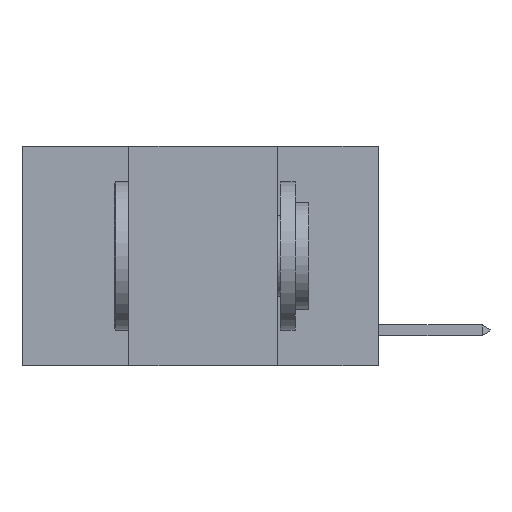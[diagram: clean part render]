
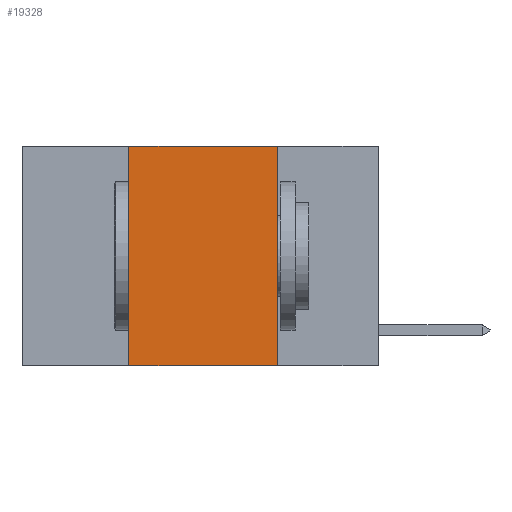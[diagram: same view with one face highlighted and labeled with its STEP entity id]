
A CAD part, left-side view. The second image highlights one B-rep face of the part: STEP entity #19328.
In plain terms, the highlighted planar face has unit normal (-1, 0, 0).
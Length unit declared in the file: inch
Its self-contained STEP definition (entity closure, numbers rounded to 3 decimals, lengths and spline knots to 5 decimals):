
#16 = EDGE_LOOP ( 'NONE', ( #15866, #12342, #7933, #7472 ) ) ;
#1249 = VECTOR ( 'NONE', #18999, 39.37008 ) ;
#1775 = LINE ( 'NONE', #7853, #6517 ) ;
#1973 = DIRECTION ( 'NONE',  ( 0., -1., 0. ) ) ;
#2403 = LINE ( 'NONE', #3987, #1249 ) ;
#3654 = FACE_OUTER_BOUND ( 'NONE', #16, .T. ) ;
#3766 = VERTEX_POINT ( 'NONE', #7858 ) ;
#3987 = CARTESIAN_POINT ( 'NONE',  ( 0., 0.6, 0. ) ) ;
#4887 = VERTEX_POINT ( 'NONE', #8288 ) ;
#5133 = DIRECTION ( 'NONE',  ( 0., 0., -1. ) ) ;
#5409 = DIRECTION ( 'NONE',  ( 0., 0., -1. ) ) ;
#5807 = DIRECTION ( 'NONE',  ( 0., 0., 1. ) ) ;
#6517 = VECTOR ( 'NONE', #1973, 39.37008 ) ;
#7255 = VECTOR ( 'NONE', #5807, 39.37008 ) ;
#7472 = ORIENTED_EDGE ( 'NONE', *, *, #8326, .T. ) ;
#7630 = VECTOR ( 'NONE', #5409, 39.37008 ) ;
#7853 = CARTESIAN_POINT ( 'NONE',  ( 0., 0.6, -0.37 ) ) ;
#7858 = CARTESIAN_POINT ( 'NONE',  ( 0., 0.17, -0.37 ) ) ;
#7933 = ORIENTED_EDGE ( 'NONE', *, *, #12472, .F. ) ;
#8288 = CARTESIAN_POINT ( 'NONE',  ( 0., 0.17, 0. ) ) ;
#8326 = EDGE_CURVE ( 'NONE', #10758, #3766, #1775, .T. ) ;
#8626 = LINE ( 'NONE', #11399, #7630 ) ;
#10227 = CARTESIAN_POINT ( 'NONE',  ( 0., 0.42, -0.37 ) ) ;
#10758 = VERTEX_POINT ( 'NONE', #10227 ) ;
#11399 = CARTESIAN_POINT ( 'NONE',  ( 0., 0.17, 0. ) ) ;
#12039 = EDGE_CURVE ( 'NONE', #13305, #4887, #2403, .T. ) ;
#12342 = ORIENTED_EDGE ( 'NONE', *, *, #12039, .F. ) ;
#12418 = AXIS2_PLACEMENT_3D ( 'NONE', #18662, #18762, #5133 ) ;
#12472 = EDGE_CURVE ( 'NONE', #10758, #13305, #13089, .T. ) ;
#13089 = LINE ( 'NONE', #16161, #7255 ) ;
#13305 = VERTEX_POINT ( 'NONE', #16113 ) ;
#15066 = EDGE_CURVE ( 'NONE', #4887, #3766, #8626, .T. ) ;
#15866 = ORIENTED_EDGE ( 'NONE', *, *, #15066, .F. ) ;
#16113 = CARTESIAN_POINT ( 'NONE',  ( 0., 0.42, 0. ) ) ;
#16161 = CARTESIAN_POINT ( 'NONE',  ( 0., 0.42, 0. ) ) ;
#17452 = PLANE ( 'NONE',  #12418 ) ;
#18662 = CARTESIAN_POINT ( 'NONE',  ( 0., 0.6, 0. ) ) ;
#18762 = DIRECTION ( 'NONE',  ( 1., 0., 0. ) ) ;
#18999 = DIRECTION ( 'NONE',  ( 0., -1., 0. ) ) ;
#19328 = ADVANCED_FACE ( 'NONE', ( #3654 ), #17452, .F. ) ;
